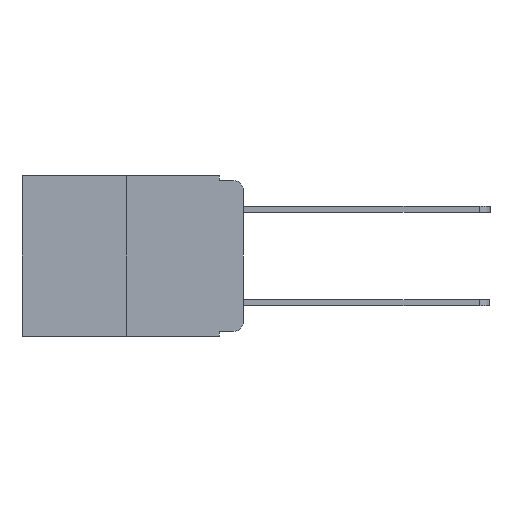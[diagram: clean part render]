
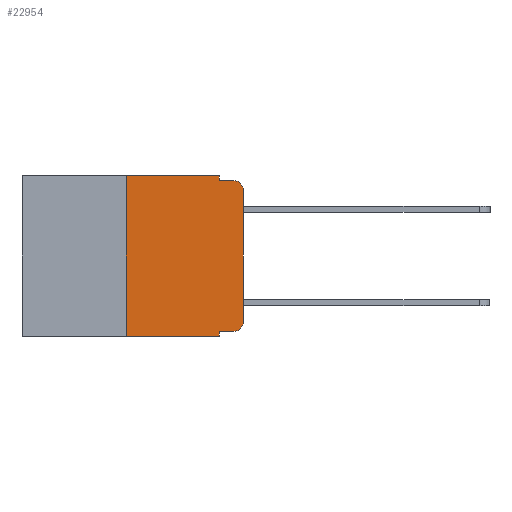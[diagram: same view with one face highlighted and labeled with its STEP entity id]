
A CAD part, left-side view. The second image highlights one B-rep face of the part: STEP entity #22954.
In plain terms, the highlighted planar face has unit normal (-1, 0, 0).
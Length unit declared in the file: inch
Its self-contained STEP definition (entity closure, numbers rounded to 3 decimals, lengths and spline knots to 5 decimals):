
#111 = VERTEX_POINT ( 'NONE', #21986 ) ;
#162 = VERTEX_POINT ( 'NONE', #19074 ) ;
#192 = VERTEX_POINT ( 'NONE', #23392 ) ;
#439 = EDGE_CURVE ( 'NONE', #111, #2995, #10752, .T. ) ;
#774 = PLANE ( 'NONE',  #13160 ) ;
#1546 = VECTOR ( 'NONE', #21145, 39.37008 ) ;
#1995 = CARTESIAN_POINT ( 'NONE',  ( 0., 0.473, 0. ) ) ;
#2221 = ORIENTED_EDGE ( 'NONE', *, *, #13077, .T. ) ;
#2234 = EDGE_CURVE ( 'NONE', #14750, #15001, #13015, .T. ) ;
#2666 = LINE ( 'NONE', #13023, #12016 ) ;
#2687 = CARTESIAN_POINT ( 'NONE',  ( 0., 0.25, -0.343 ) ) ;
#2995 = VERTEX_POINT ( 'NONE', #19513 ) ;
#3062 = VECTOR ( 'NONE', #18293, 39.37008 ) ;
#3075 = ORIENTED_EDGE ( 'NONE', *, *, #12287, .T. ) ;
#3140 = VERTEX_POINT ( 'NONE', #6819 ) ;
#3737 = CARTESIAN_POINT ( 'NONE',  ( 0., 0.02, -0.01 ) ) ;
#4594 = EDGE_LOOP ( 'NONE', ( #16537, #3075, #7938, #7744, #7660, #22437, #22881, #12996, #20558, #2221 ) ) ;
#4688 = DIRECTION ( 'NONE',  ( 0., 0., -1. ) ) ;
#4692 = CARTESIAN_POINT ( 'NONE',  ( 0., 0.473, -0.343 ) ) ;
#4694 = CARTESIAN_POINT ( 'NONE',  ( 0., 0.02, -0.03 ) ) ;
#5864 = VECTOR ( 'NONE', #19754, 39.37008 ) ;
#6584 = DIRECTION ( 'NONE',  ( 0., 0., -1. ) ) ;
#6819 = CARTESIAN_POINT ( 'NONE',  ( 0., 0.051, -0.01 ) ) ;
#7460 = DIRECTION ( 'NONE',  ( 0., -1., 0. ) ) ;
#7660 = ORIENTED_EDGE ( 'NONE', *, *, #11326, .F. ) ;
#7744 = ORIENTED_EDGE ( 'NONE', *, *, #18410, .F. ) ;
#7938 = ORIENTED_EDGE ( 'NONE', *, *, #14777, .F. ) ;
#8005 = VERTEX_POINT ( 'NONE', #16202 ) ;
#8170 = CIRCLE ( 'NONE', #23664, 0.02 ) ;
#9046 = CARTESIAN_POINT ( 'NONE',  ( 0., 0.02, -0.313 ) ) ;
#9582 = DIRECTION ( 'NONE',  ( 0., -1., 0. ) ) ;
#10246 = CIRCLE ( 'NONE', #19791, 0.02 ) ;
#10572 = EDGE_CURVE ( 'NONE', #111, #162, #2666, .T. ) ;
#10752 = LINE ( 'NONE', #22989, #5864 ) ;
#10874 = DIRECTION ( 'NONE',  ( 0., 0., -1. ) ) ;
#11106 = CARTESIAN_POINT ( 'NONE',  ( 0., 0., 0. ) ) ;
#11326 = EDGE_CURVE ( 'NONE', #8005, #192, #20778, .T. ) ;
#11344 = FACE_OUTER_BOUND ( 'NONE', #4594, .T. ) ;
#11826 = CARTESIAN_POINT ( 'NONE',  ( 0., 0.25, 0. ) ) ;
#11890 = VECTOR ( 'NONE', #15857, 39.37008 ) ;
#12016 = VECTOR ( 'NONE', #7460, 39.37008 ) ;
#12287 = EDGE_CURVE ( 'NONE', #15001, #12649, #10246, .T. ) ;
#12471 = LINE ( 'NONE', #11826, #16789 ) ;
#12566 = LINE ( 'NONE', #22700, #13156 ) ;
#12649 = VERTEX_POINT ( 'NONE', #3737 ) ;
#12996 = ORIENTED_EDGE ( 'NONE', *, *, #439, .F. ) ;
#13015 = LINE ( 'NONE', #11106, #3062 ) ;
#13023 = CARTESIAN_POINT ( 'NONE',  ( 0., 0.051, -0.333 ) ) ;
#13077 = EDGE_CURVE ( 'NONE', #162, #14750, #8170, .T. ) ;
#13156 = VECTOR ( 'NONE', #17396, 39.37008 ) ;
#13160 = AXIS2_PLACEMENT_3D ( 'NONE', #13920, #15781, #4688 ) ;
#13920 = CARTESIAN_POINT ( 'NONE',  ( 0., 0.473, 0. ) ) ;
#14545 = CARTESIAN_POINT ( 'NONE',  ( 0., 0., -0.03 ) ) ;
#14750 = VERTEX_POINT ( 'NONE', #19263 ) ;
#14777 = EDGE_CURVE ( 'NONE', #3140, #12649, #16452, .T. ) ;
#15001 = VERTEX_POINT ( 'NONE', #14545 ) ;
#15465 = VERTEX_POINT ( 'NONE', #2687 ) ;
#15572 = DIRECTION ( 'NONE',  ( 0., 0., 1. ) ) ;
#15781 = DIRECTION ( 'NONE',  ( 1., 0., 0. ) ) ;
#15857 = DIRECTION ( 'NONE',  ( 0., -1., 0. ) ) ;
#16043 = VECTOR ( 'NONE', #9582, 39.37008 ) ;
#16202 = CARTESIAN_POINT ( 'NONE',  ( 0., 0.25, 0. ) ) ;
#16452 = LINE ( 'NONE', #19341, #1546 ) ;
#16537 = ORIENTED_EDGE ( 'NONE', *, *, #2234, .T. ) ;
#16789 = VECTOR ( 'NONE', #15572, 39.37008 ) ;
#17351 = LINE ( 'NONE', #4692, #11890 ) ;
#17396 = DIRECTION ( 'NONE',  ( 0., 0., -1. ) ) ;
#17589 = DIRECTION ( 'NONE',  ( -1., 0., 0. ) ) ;
#18293 = DIRECTION ( 'NONE',  ( 0., 0., 1. ) ) ;
#18410 = EDGE_CURVE ( 'NONE', #192, #3140, #12566, .T. ) ;
#19074 = CARTESIAN_POINT ( 'NONE',  ( 0., 0.02, -0.333 ) ) ;
#19263 = CARTESIAN_POINT ( 'NONE',  ( 0., 0., -0.313 ) ) ;
#19341 = CARTESIAN_POINT ( 'NONE',  ( 0., 0.051, -0.01 ) ) ;
#19513 = CARTESIAN_POINT ( 'NONE',  ( 0., 0.051, -0.343 ) ) ;
#19722 = EDGE_CURVE ( 'NONE', #15465, #2995, #17351, .T. ) ;
#19754 = DIRECTION ( 'NONE',  ( 0., 0., -1. ) ) ;
#19791 = AXIS2_PLACEMENT_3D ( 'NONE', #4694, #17589, #6584 ) ;
#20558 = ORIENTED_EDGE ( 'NONE', *, *, #10572, .T. ) ;
#20778 = LINE ( 'NONE', #1995, #16043 ) ;
#20781 = EDGE_CURVE ( 'NONE', #15465, #8005, #12471, .T. ) ;
#21145 = DIRECTION ( 'NONE',  ( 0., -1., 0. ) ) ;
#21756 = DIRECTION ( 'NONE',  ( -1., 0., 0. ) ) ;
#21986 = CARTESIAN_POINT ( 'NONE',  ( 0., 0.051, -0.333 ) ) ;
#22437 = ORIENTED_EDGE ( 'NONE', *, *, #20781, .F. ) ;
#22700 = CARTESIAN_POINT ( 'NONE',  ( 0., 0.051, 0. ) ) ;
#22881 = ORIENTED_EDGE ( 'NONE', *, *, #19722, .T. ) ;
#22954 = ADVANCED_FACE ( 'NONE', ( #11344 ), #774, .F. ) ;
#22989 = CARTESIAN_POINT ( 'NONE',  ( 0., 0.051, 0. ) ) ;
#23392 = CARTESIAN_POINT ( 'NONE',  ( 0., 0.051, 0. ) ) ;
#23664 = AXIS2_PLACEMENT_3D ( 'NONE', #9046, #21756, #10874 ) ;
